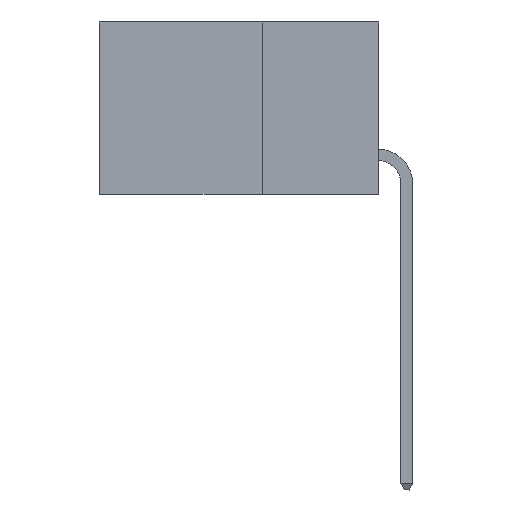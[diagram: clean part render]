
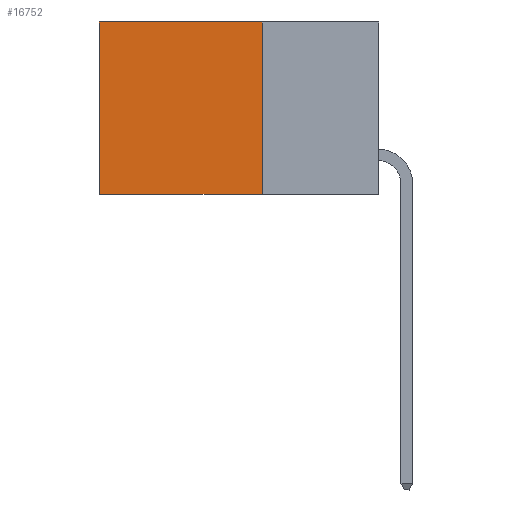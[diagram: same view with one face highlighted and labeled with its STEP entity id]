
A CAD part, left-side view. The second image highlights one B-rep face of the part: STEP entity #16752.
In plain terms, the highlighted planar face has unit normal (-1, 0, 0).
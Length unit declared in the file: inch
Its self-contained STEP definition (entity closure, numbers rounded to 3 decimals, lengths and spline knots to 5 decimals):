
#736 = VERTEX_POINT ( 'NONE', #21133 ) ;
#840 = CARTESIAN_POINT ( 'NONE',  ( 0.298, 0.25, 0. ) ) ;
#2288 = ORIENTED_EDGE ( 'NONE', *, *, #28555, .T. ) ;
#2705 = CARTESIAN_POINT ( 'NONE',  ( 0.298, 0.6, 0. ) ) ;
#3201 = DIRECTION ( 'NONE',  ( 0., 0., -1. ) ) ;
#3660 = DIRECTION ( 'NONE',  ( 0., 1., 0. ) ) ;
#3962 = EDGE_CURVE ( 'NONE', #4653, #9882, #14265, .T. ) ;
#4093 = VECTOR ( 'NONE', #12090, 39.37008 ) ;
#4367 = EDGE_CURVE ( 'NONE', #20745, #9882, #27937, .T. ) ;
#4653 = VERTEX_POINT ( 'NONE', #29083 ) ;
#6179 = AXIS2_PLACEMENT_3D ( 'NONE', #840, #17191, #3201 ) ;
#6948 = ORIENTED_EDGE ( 'NONE', *, *, #4367, .T. ) ;
#7869 = PLANE ( 'NONE',  #6179 ) ;
#8087 = VECTOR ( 'NONE', #3660, 39.37008 ) ;
#8768 = VECTOR ( 'NONE', #21405, 39.37008 ) ;
#9882 = VERTEX_POINT ( 'NONE', #14817 ) ;
#10694 = ORIENTED_EDGE ( 'NONE', *, *, #14494, .F. ) ;
#12090 = DIRECTION ( 'NONE',  ( 0., 1., 0. ) ) ;
#14265 = LINE ( 'NONE', #26829, #8087 ) ;
#14494 = EDGE_CURVE ( 'NONE', #736, #4653, #21169, .T. ) ;
#14817 = CARTESIAN_POINT ( 'NONE',  ( 0.298, 0.6, -0.37 ) ) ;
#16090 = ORIENTED_EDGE ( 'NONE', *, *, #3962, .F. ) ;
#16513 = LINE ( 'NONE', #28215, #4093 ) ;
#16752 = ADVANCED_FACE ( 'NONE', ( #21097 ), #7869, .F. ) ;
#17110 = DIRECTION ( 'NONE',  ( 0., 0., -1. ) ) ;
#17191 = DIRECTION ( 'NONE',  ( 1., 0., 0. ) ) ;
#20679 = CARTESIAN_POINT ( 'NONE',  ( 0.298, 0.6, 0. ) ) ;
#20745 = VERTEX_POINT ( 'NONE', #20679 ) ;
#21097 = FACE_OUTER_BOUND ( 'NONE', #21385, .T. ) ;
#21133 = CARTESIAN_POINT ( 'NONE',  ( 0.298, 0.25, 0. ) ) ;
#21169 = LINE ( 'NONE', #28593, #27270 ) ;
#21385 = EDGE_LOOP ( 'NONE', ( #6948, #16090, #10694, #2288 ) ) ;
#21405 = DIRECTION ( 'NONE',  ( 0., 0., -1. ) ) ;
#26829 = CARTESIAN_POINT ( 'NONE',  ( 0.298, 0.25, -0.37 ) ) ;
#27270 = VECTOR ( 'NONE', #17110, 39.37008 ) ;
#27937 = LINE ( 'NONE', #2705, #8768 ) ;
#28215 = CARTESIAN_POINT ( 'NONE',  ( 0.298, 0.25, 0. ) ) ;
#28555 = EDGE_CURVE ( 'NONE', #736, #20745, #16513, .T. ) ;
#28593 = CARTESIAN_POINT ( 'NONE',  ( 0.298, 0.25, 0. ) ) ;
#29083 = CARTESIAN_POINT ( 'NONE',  ( 0.298, 0.25, -0.37 ) ) ;
